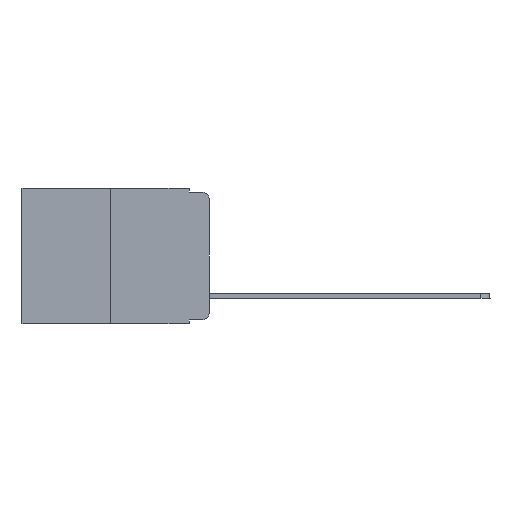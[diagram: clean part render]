
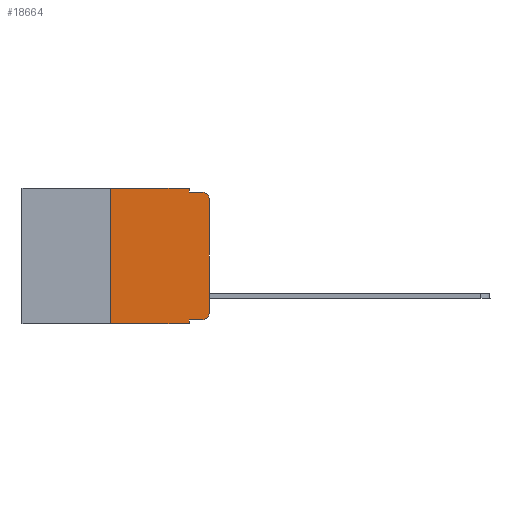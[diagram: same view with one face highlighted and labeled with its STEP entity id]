
A CAD part, left-side view. The second image highlights one B-rep face of the part: STEP entity #18664.
In plain terms, the highlighted planar face has unit normal (-1, 0, 0).
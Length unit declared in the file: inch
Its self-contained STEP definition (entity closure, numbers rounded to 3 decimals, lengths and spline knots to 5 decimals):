
#81 = LINE ( 'NONE', #11471, #10133 ) ;
#172 = EDGE_CURVE ( 'NONE', #10431, #16106, #81, .T. ) ;
#211 = LINE ( 'NONE', #13279, #10029 ) ;
#312 = CARTESIAN_POINT ( 'NONE',  ( 0., 0.02, -0.313 ) ) ;
#601 = ORIENTED_EDGE ( 'NONE', *, *, #4337, .T. ) ;
#1128 = ORIENTED_EDGE ( 'NONE', *, *, #6098, .F. ) ;
#1152 = VERTEX_POINT ( 'NONE', #6133 ) ;
#1227 = ORIENTED_EDGE ( 'NONE', *, *, #2549, .F. ) ;
#1327 = VECTOR ( 'NONE', #5592, 39.37008 ) ;
#1833 = LINE ( 'NONE', #17407, #14055 ) ;
#2216 = EDGE_CURVE ( 'NONE', #10431, #11551, #8401, .T. ) ;
#2264 = EDGE_CURVE ( 'NONE', #5382, #11572, #8624, .T. ) ;
#2355 = LINE ( 'NONE', #19606, #8365 ) ;
#2549 = EDGE_CURVE ( 'NONE', #1152, #11572, #211, .T. ) ;
#2589 = DIRECTION ( 'NONE',  ( 0., 0., -1. ) ) ;
#3463 = ORIENTED_EDGE ( 'NONE', *, *, #2216, .F. ) ;
#3509 = VERTEX_POINT ( 'NONE', #9324 ) ;
#3853 = VECTOR ( 'NONE', #2589, 39.37008 ) ;
#4175 = DIRECTION ( 'NONE',  ( 1., 0., 0. ) ) ;
#4237 = PLANE ( 'NONE',  #5573 ) ;
#4277 = CARTESIAN_POINT ( 'NONE',  ( 0., 0., -0.313 ) ) ;
#4337 = EDGE_CURVE ( 'NONE', #16106, #19404, #10954, .T. ) ;
#5282 = LINE ( 'NONE', #8182, #7912 ) ;
#5367 = VERTEX_POINT ( 'NONE', #7909 ) ;
#5382 = VERTEX_POINT ( 'NONE', #12322 ) ;
#5399 = CARTESIAN_POINT ( 'NONE',  ( 0., 0.051, -0.333 ) ) ;
#5573 = AXIS2_PLACEMENT_3D ( 'NONE', #13387, #4175, #5664 ) ;
#5592 = DIRECTION ( 'NONE',  ( 0., 0., -1. ) ) ;
#5664 = DIRECTION ( 'NONE',  ( 0., 0., -1. ) ) ;
#6098 = EDGE_CURVE ( 'NONE', #9593, #5367, #5282, .T. ) ;
#6133 = CARTESIAN_POINT ( 'NONE',  ( 0., 0.051, -0.01 ) ) ;
#6877 = ORIENTED_EDGE ( 'NONE', *, *, #2264, .T. ) ;
#7089 = EDGE_CURVE ( 'NONE', #3509, #9593, #8836, .T. ) ;
#7143 = VECTOR ( 'NONE', #8208, 39.37008 ) ;
#7368 = EDGE_CURVE ( 'NONE', #19404, #5382, #2355, .T. ) ;
#7633 = EDGE_LOOP ( 'NONE', ( #18258, #6877, #1227, #8812, #1128, #19123, #9880, #3463, #13032, #601 ) ) ;
#7909 = CARTESIAN_POINT ( 'NONE',  ( 0., 0.051, 0. ) ) ;
#7912 = VECTOR ( 'NONE', #9692, 39.37008 ) ;
#8112 = EDGE_CURVE ( 'NONE', #3509, #11551, #1833, .T. ) ;
#8182 = CARTESIAN_POINT ( 'NONE',  ( 0., 0.473, 0. ) ) ;
#8208 = DIRECTION ( 'NONE',  ( 0., 0., 1. ) ) ;
#8310 = DIRECTION ( 'NONE',  ( 0., 0., 1. ) ) ;
#8335 = LINE ( 'NONE', #19478, #1327 ) ;
#8365 = VECTOR ( 'NONE', #8310, 39.37008 ) ;
#8382 = DIRECTION ( 'NONE',  ( 0., -1., 0. ) ) ;
#8401 = LINE ( 'NONE', #11753, #3853 ) ;
#8414 = DIRECTION ( 'NONE',  ( 0., -1., 0. ) ) ;
#8624 = CIRCLE ( 'NONE', #11858, 0.02 ) ;
#8812 = ORIENTED_EDGE ( 'NONE', *, *, #14725, .F. ) ;
#8836 = LINE ( 'NONE', #17358, #7143 ) ;
#9324 = CARTESIAN_POINT ( 'NONE',  ( 0., 0.25, -0.343 ) ) ;
#9593 = VERTEX_POINT ( 'NONE', #12395 ) ;
#9692 = DIRECTION ( 'NONE',  ( 0., -1., 0. ) ) ;
#9880 = ORIENTED_EDGE ( 'NONE', *, *, #8112, .T. ) ;
#10029 = VECTOR ( 'NONE', #19381, 39.37008 ) ;
#10065 = CARTESIAN_POINT ( 'NONE',  ( 0., 0.051, -0.343 ) ) ;
#10133 = VECTOR ( 'NONE', #8414, 39.37008 ) ;
#10285 = FACE_OUTER_BOUND ( 'NONE', #7633, .T. ) ;
#10431 = VERTEX_POINT ( 'NONE', #5399 ) ;
#10807 = DIRECTION ( 'NONE',  ( -1., 0., 0. ) ) ;
#10954 = CIRCLE ( 'NONE', #18226, 0.02 ) ;
#11471 = CARTESIAN_POINT ( 'NONE',  ( 0., 0.051, -0.333 ) ) ;
#11551 = VERTEX_POINT ( 'NONE', #10065 ) ;
#11572 = VERTEX_POINT ( 'NONE', #17841 ) ;
#11753 = CARTESIAN_POINT ( 'NONE',  ( 0., 0.051, 0. ) ) ;
#11858 = AXIS2_PLACEMENT_3D ( 'NONE', #15082, #19719, #12090 ) ;
#12090 = DIRECTION ( 'NONE',  ( 0., 0., -1. ) ) ;
#12322 = CARTESIAN_POINT ( 'NONE',  ( 0., 0., -0.03 ) ) ;
#12395 = CARTESIAN_POINT ( 'NONE',  ( 0., 0.25, 0. ) ) ;
#13032 = ORIENTED_EDGE ( 'NONE', *, *, #172, .T. ) ;
#13279 = CARTESIAN_POINT ( 'NONE',  ( 0., 0.051, -0.01 ) ) ;
#13387 = CARTESIAN_POINT ( 'NONE',  ( 0., 0.473, 0. ) ) ;
#14055 = VECTOR ( 'NONE', #8382, 39.37008 ) ;
#14725 = EDGE_CURVE ( 'NONE', #5367, #1152, #8335, .T. ) ;
#15082 = CARTESIAN_POINT ( 'NONE',  ( 0., 0.02, -0.03 ) ) ;
#16106 = VERTEX_POINT ( 'NONE', #16599 ) ;
#16599 = CARTESIAN_POINT ( 'NONE',  ( 0., 0.02, -0.333 ) ) ;
#17358 = CARTESIAN_POINT ( 'NONE',  ( 0., 0.25, 0. ) ) ;
#17407 = CARTESIAN_POINT ( 'NONE',  ( 0., 0.473, -0.343 ) ) ;
#17841 = CARTESIAN_POINT ( 'NONE',  ( 0., 0.02, -0.01 ) ) ;
#18226 = AXIS2_PLACEMENT_3D ( 'NONE', #312, #10807, #18641 ) ;
#18258 = ORIENTED_EDGE ( 'NONE', *, *, #7368, .T. ) ;
#18641 = DIRECTION ( 'NONE',  ( 0., 0., -1. ) ) ;
#18664 = ADVANCED_FACE ( 'NONE', ( #10285 ), #4237, .F. ) ;
#19123 = ORIENTED_EDGE ( 'NONE', *, *, #7089, .F. ) ;
#19381 = DIRECTION ( 'NONE',  ( 0., -1., 0. ) ) ;
#19404 = VERTEX_POINT ( 'NONE', #4277 ) ;
#19478 = CARTESIAN_POINT ( 'NONE',  ( 0., 0.051, 0. ) ) ;
#19606 = CARTESIAN_POINT ( 'NONE',  ( 0., 0., 0. ) ) ;
#19719 = DIRECTION ( 'NONE',  ( -1., 0., 0. ) ) ;
